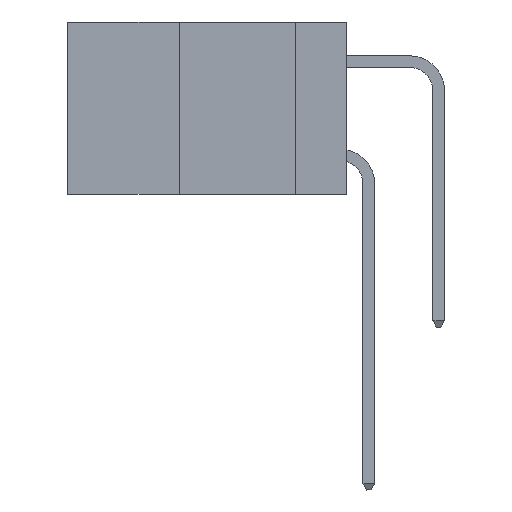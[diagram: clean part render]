
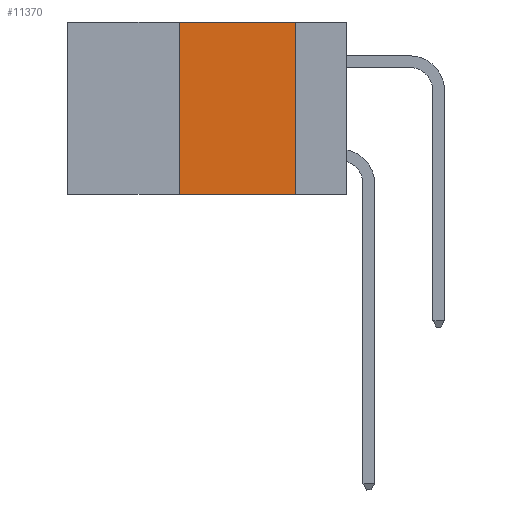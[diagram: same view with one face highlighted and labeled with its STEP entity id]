
A CAD part, left-side view. The second image highlights one B-rep face of the part: STEP entity #11370.
In plain terms, the highlighted planar face has unit normal (-1, 0, 0).
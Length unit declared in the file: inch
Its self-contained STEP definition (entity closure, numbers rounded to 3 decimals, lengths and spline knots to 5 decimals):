
#241 = CARTESIAN_POINT ( 'NONE',  ( 0., 0.6, -0.37 ) ) ;
#657 = CARTESIAN_POINT ( 'NONE',  ( 0., 0.36, 0. ) ) ;
#745 = EDGE_CURVE ( 'NONE', #4964, #13951, #14665, .T. ) ;
#1059 = CARTESIAN_POINT ( 'NONE',  ( 0., 0.6, 0. ) ) ;
#1465 = EDGE_LOOP ( 'NONE', ( #3045, #3104, #3642, #3785 ) ) ;
#1667 = PLANE ( 'NONE',  #9726 ) ;
#1936 = VECTOR ( 'NONE', #8733, 39.37008 ) ;
#2289 = EDGE_CURVE ( 'NONE', #4964, #10897, #5020, .T. ) ;
#2817 = DIRECTION ( 'NONE',  ( 1., 0., 0. ) ) ;
#3045 = ORIENTED_EDGE ( 'NONE', *, *, #9496, .F. ) ;
#3104 = ORIENTED_EDGE ( 'NONE', *, *, #12888, .F. ) ;
#3642 = ORIENTED_EDGE ( 'NONE', *, *, #745, .F. ) ;
#3785 = ORIENTED_EDGE ( 'NONE', *, *, #2289, .T. ) ;
#4000 = CARTESIAN_POINT ( 'NONE',  ( 0., 0.36, -0.37 ) ) ;
#4150 = VECTOR ( 'NONE', #7007, 39.37008 ) ;
#4537 = LINE ( 'NONE', #1059, #4150 ) ;
#4964 = VERTEX_POINT ( 'NONE', #4000 ) ;
#5020 = LINE ( 'NONE', #241, #8246 ) ;
#5406 = CARTESIAN_POINT ( 'NONE',  ( 0., 0.11, 0. ) ) ;
#6160 = DIRECTION ( 'NONE',  ( 0., 0., 1. ) ) ;
#6902 = CARTESIAN_POINT ( 'NONE',  ( 0., 0.36, 0. ) ) ;
#7007 = DIRECTION ( 'NONE',  ( 0., -1., 0. ) ) ;
#7516 = CARTESIAN_POINT ( 'NONE',  ( 0., 0.11, 0. ) ) ;
#8246 = VECTOR ( 'NONE', #10979, 39.37008 ) ;
#8327 = LINE ( 'NONE', #7516, #1936 ) ;
#8733 = DIRECTION ( 'NONE',  ( 0., 0., -1. ) ) ;
#8827 = CARTESIAN_POINT ( 'NONE',  ( 0., 0.6, 0. ) ) ;
#8843 = VECTOR ( 'NONE', #6160, 39.37008 ) ;
#9496 = EDGE_CURVE ( 'NONE', #11509, #10897, #8327, .T. ) ;
#9726 = AXIS2_PLACEMENT_3D ( 'NONE', #8827, #2817, #11189 ) ;
#10897 = VERTEX_POINT ( 'NONE', #12700 ) ;
#10979 = DIRECTION ( 'NONE',  ( 0., -1., 0. ) ) ;
#11189 = DIRECTION ( 'NONE',  ( 0., 0., -1. ) ) ;
#11370 = ADVANCED_FACE ( 'NONE', ( #11591 ), #1667, .F. ) ;
#11509 = VERTEX_POINT ( 'NONE', #5406 ) ;
#11591 = FACE_OUTER_BOUND ( 'NONE', #1465, .T. ) ;
#12700 = CARTESIAN_POINT ( 'NONE',  ( 0., 0.11, -0.37 ) ) ;
#12888 = EDGE_CURVE ( 'NONE', #13951, #11509, #4537, .T. ) ;
#13951 = VERTEX_POINT ( 'NONE', #657 ) ;
#14665 = LINE ( 'NONE', #6902, #8843 ) ;
